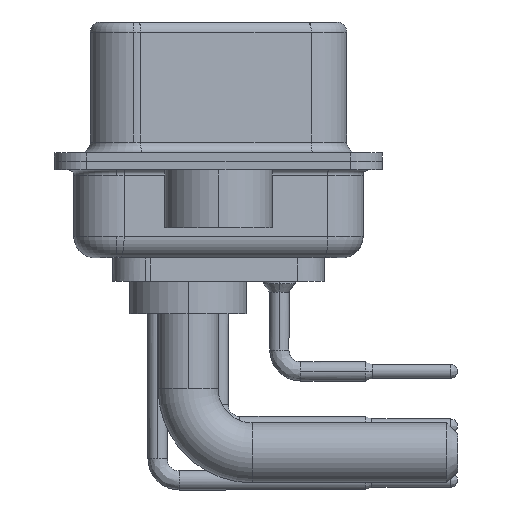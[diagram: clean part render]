
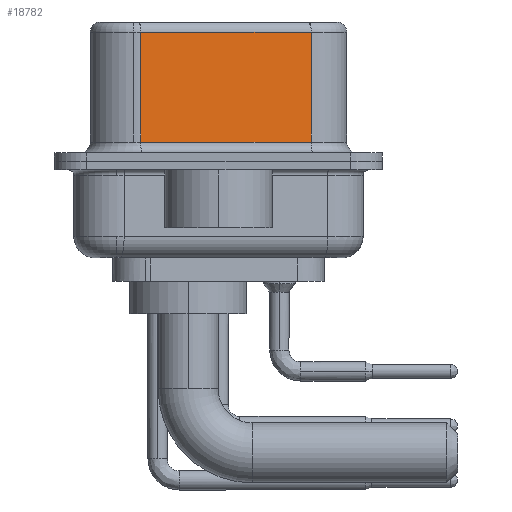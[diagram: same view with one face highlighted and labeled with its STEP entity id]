
A CAD part, left-side view. The second image highlights one B-rep face of the part: STEP entity #18782.
In plain terms, the highlighted planar face has unit normal (-0.985, -0.174, 0).
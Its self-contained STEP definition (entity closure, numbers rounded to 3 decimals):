
#245 = EDGE_LOOP ( 'NONE', ( #14962, #22645, #22904, #4624 ) ) ;
#2199 = CARTESIAN_POINT ( 'NONE',  ( 5.132, -4.322, 6.52 ) ) ;
#2363 = EDGE_CURVE ( 'NONE', #19616, #15802, #31715, .T. ) ;
#4040 = CARTESIAN_POINT ( 'NONE',  ( 5.132, -4.322, 6.52 ) ) ;
#4467 = DIRECTION ( 'NONE',  ( 0.174, -0.985, 0. ) ) ;
#4624 = ORIENTED_EDGE ( 'NONE', *, *, #27910, .T. ) ;
#4730 = VECTOR ( 'NONE', #7791, 1000. ) ;
#6384 = CARTESIAN_POINT ( 'NONE',  ( 5.132, -4.322, 6.02 ) ) ;
#6457 = DIRECTION ( 'NONE',  ( 0.985, 0.174, 0. ) ) ;
#7566 = LINE ( 'NONE', #12921, #8764 ) ;
#7639 = DIRECTION ( 'NONE',  ( -0.174, 0.985, 0. ) ) ;
#7791 = DIRECTION ( 'NONE',  ( 0., 0., -1. ) ) ;
#8680 = EDGE_CURVE ( 'NONE', #19017, #19616, #18386, .T. ) ;
#8764 = VECTOR ( 'NONE', #4467, 1000. ) ;
#10559 = CARTESIAN_POINT ( 'NONE',  ( 3.73, 3.628, 6.52 ) ) ;
#10585 = CARTESIAN_POINT ( 'NONE',  ( 5.132, -4.322, 6.02 ) ) ;
#10639 = CARTESIAN_POINT ( 'NONE',  ( 5.132, -4.322, 0.9 ) ) ;
#12216 = CARTESIAN_POINT ( 'NONE',  ( 3.73, 3.628, 6.02 ) ) ;
#12753 = DIRECTION ( 'NONE',  ( 0., 0., -1. ) ) ;
#12921 = CARTESIAN_POINT ( 'NONE',  ( 5.132, -4.322, 0.9 ) ) ;
#14942 = FACE_OUTER_BOUND ( 'NONE', #245, .T. ) ;
#14962 = ORIENTED_EDGE ( 'NONE', *, *, #33647, .F. ) ;
#15802 = VERTEX_POINT ( 'NONE', #32864 ) ;
#16077 = VERTEX_POINT ( 'NONE', #10639 ) ;
#16892 = VECTOR ( 'NONE', #7639, 1000. ) ;
#18386 = LINE ( 'NONE', #10585, #16892 ) ;
#18782 = ADVANCED_FACE ( 'NONE', ( #14942 ), #27794, .F. ) ;
#19017 = VERTEX_POINT ( 'NONE', #6384 ) ;
#19616 = VERTEX_POINT ( 'NONE', #12216 ) ;
#22634 = VECTOR ( 'NONE', #12753, 1000. ) ;
#22645 = ORIENTED_EDGE ( 'NONE', *, *, #8680, .T. ) ;
#22904 = ORIENTED_EDGE ( 'NONE', *, *, #2363, .T. ) ;
#25952 = LINE ( 'NONE', #2199, #22634 ) ;
#27794 = PLANE ( 'NONE',  #34031 ) ;
#27910 = EDGE_CURVE ( 'NONE', #15802, #16077, #7566, .T. ) ;
#30562 = DIRECTION ( 'NONE',  ( -0.174, 0.985, 0. ) ) ;
#31715 = LINE ( 'NONE', #10559, #4730 ) ;
#32864 = CARTESIAN_POINT ( 'NONE',  ( 3.73, 3.628, 0.9 ) ) ;
#33647 = EDGE_CURVE ( 'NONE', #19017, #16077, #25952, .T. ) ;
#34031 = AXIS2_PLACEMENT_3D ( 'NONE', #4040, #6457, #30562 ) ;
